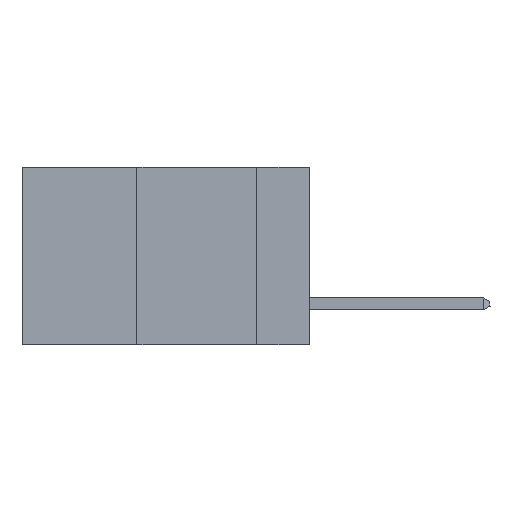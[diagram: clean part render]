
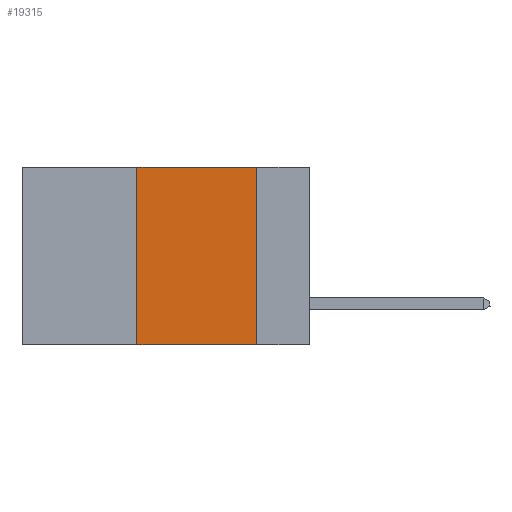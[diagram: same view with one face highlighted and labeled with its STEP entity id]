
A CAD part, left-side view. The second image highlights one B-rep face of the part: STEP entity #19315.
In plain terms, the highlighted planar face has unit normal (-1, 0, 0).
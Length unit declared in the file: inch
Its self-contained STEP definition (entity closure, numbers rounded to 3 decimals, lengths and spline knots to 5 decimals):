
#761 = CARTESIAN_POINT ( 'NONE',  ( 0., 0.36, 0. ) ) ;
#2963 = CARTESIAN_POINT ( 'NONE',  ( 0., 0.6, 0. ) ) ;
#3400 = DIRECTION ( 'NONE',  ( 0., 0., 1. ) ) ;
#3998 = VECTOR ( 'NONE', #3400, 39.37008 ) ;
#4728 = FACE_OUTER_BOUND ( 'NONE', #35597, .T. ) ;
#5047 = VECTOR ( 'NONE', #40395, 39.37008 ) ;
#5683 = CARTESIAN_POINT ( 'NONE',  ( 0., 0.11, 0. ) ) ;
#7969 = LINE ( 'NONE', #25435, #5047 ) ;
#9100 = VERTEX_POINT ( 'NONE', #36008 ) ;
#12310 = VECTOR ( 'NONE', #16930, 39.37008 ) ;
#13536 = CARTESIAN_POINT ( 'NONE',  ( 0., 0.11, -0.37 ) ) ;
#13539 = CARTESIAN_POINT ( 'NONE',  ( 0., 0.11, 0. ) ) ;
#14078 = AXIS2_PLACEMENT_3D ( 'NONE', #2963, #44248, #40048 ) ;
#14574 = EDGE_CURVE ( 'NONE', #9100, #22110, #34078, .T. ) ;
#15136 = LINE ( 'NONE', #45007, #3998 ) ;
#16569 = EDGE_CURVE ( 'NONE', #18524, #22110, #44954, .T. ) ;
#16930 = DIRECTION ( 'NONE',  ( 0., 0., -1. ) ) ;
#17976 = ORIENTED_EDGE ( 'NONE', *, *, #14574, .T. ) ;
#18524 = VERTEX_POINT ( 'NONE', #13539 ) ;
#19315 = ADVANCED_FACE ( 'NONE', ( #4728 ), #48156, .F. ) ;
#22110 = VERTEX_POINT ( 'NONE', #13536 ) ;
#24187 = VECTOR ( 'NONE', #33232, 39.37008 ) ;
#25435 = CARTESIAN_POINT ( 'NONE',  ( 0., 0.6, 0. ) ) ;
#26369 = CARTESIAN_POINT ( 'NONE',  ( 0., 0.6, -0.37 ) ) ;
#31694 = ORIENTED_EDGE ( 'NONE', *, *, #35873, .F. ) ;
#33232 = DIRECTION ( 'NONE',  ( 0., -1., 0. ) ) ;
#34078 = LINE ( 'NONE', #26369, #24187 ) ;
#35597 = EDGE_LOOP ( 'NONE', ( #37751, #35901, #31694, #17976 ) ) ;
#35873 = EDGE_CURVE ( 'NONE', #9100, #40998, #15136, .T. ) ;
#35901 = ORIENTED_EDGE ( 'NONE', *, *, #48108, .F. ) ;
#36008 = CARTESIAN_POINT ( 'NONE',  ( 0., 0.36, -0.37 ) ) ;
#37751 = ORIENTED_EDGE ( 'NONE', *, *, #16569, .F. ) ;
#40048 = DIRECTION ( 'NONE',  ( 0., 0., -1. ) ) ;
#40395 = DIRECTION ( 'NONE',  ( 0., -1., 0. ) ) ;
#40998 = VERTEX_POINT ( 'NONE', #761 ) ;
#44248 = DIRECTION ( 'NONE',  ( 1., 0., 0. ) ) ;
#44954 = LINE ( 'NONE', #5683, #12310 ) ;
#45007 = CARTESIAN_POINT ( 'NONE',  ( 0., 0.36, 0. ) ) ;
#48108 = EDGE_CURVE ( 'NONE', #40998, #18524, #7969, .T. ) ;
#48156 = PLANE ( 'NONE',  #14078 ) ;
